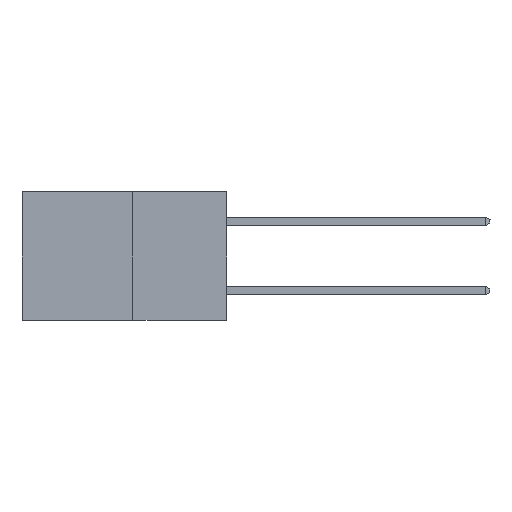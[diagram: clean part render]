
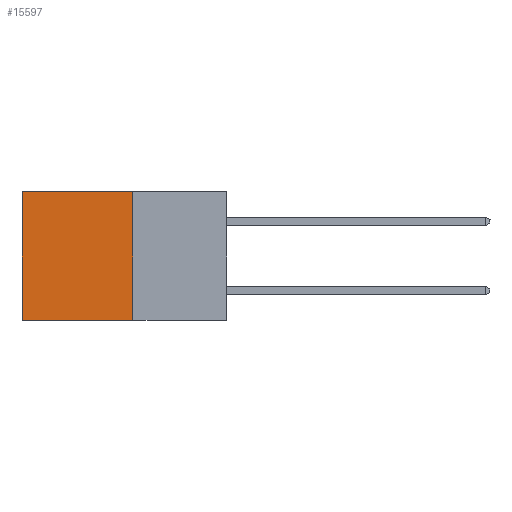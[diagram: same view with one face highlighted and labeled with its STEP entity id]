
A CAD part, left-side view. The second image highlights one B-rep face of the part: STEP entity #15597.
In plain terms, the highlighted planar face has unit normal (-1, 0, 0).
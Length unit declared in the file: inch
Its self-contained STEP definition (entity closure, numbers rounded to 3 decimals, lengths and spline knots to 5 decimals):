
#1082 = DIRECTION ( 'NONE',  ( 0., 1., 0. ) ) ;
#4852 = CARTESIAN_POINT ( 'NONE',  ( 0.277, 0.27, -0.37 ) ) ;
#4977 = CARTESIAN_POINT ( 'NONE',  ( 0.277, 0.27, -0.37 ) ) ;
#6089 = PLANE ( 'NONE',  #22583 ) ;
#6688 = VERTEX_POINT ( 'NONE', #24972 ) ;
#7414 = EDGE_CURVE ( 'NONE', #6688, #21558, #27898, .T. ) ;
#8300 = DIRECTION ( 'NONE',  ( 1., 0., 0. ) ) ;
#8343 = ORIENTED_EDGE ( 'NONE', *, *, #7414, .T. ) ;
#8910 = VECTOR ( 'NONE', #13236, 39.37008 ) ;
#9959 = EDGE_CURVE ( 'NONE', #21558, #11272, #15462, .T. ) ;
#11272 = VERTEX_POINT ( 'NONE', #15071 ) ;
#11439 = EDGE_CURVE ( 'NONE', #6688, #18386, #11996, .T. ) ;
#11572 = CARTESIAN_POINT ( 'NONE',  ( 0.277, 0.59, 0. ) ) ;
#11648 = DIRECTION ( 'NONE',  ( 0., 0., -1. ) ) ;
#11996 = LINE ( 'NONE', #4852, #17097 ) ;
#13236 = DIRECTION ( 'NONE',  ( 0., 0., -1. ) ) ;
#14269 = ORIENTED_EDGE ( 'NONE', *, *, #11439, .F. ) ;
#15071 = CARTESIAN_POINT ( 'NONE',  ( 0.277, 0.59, -0.37 ) ) ;
#15462 = LINE ( 'NONE', #24146, #8910 ) ;
#15550 = LINE ( 'NONE', #4977, #27225 ) ;
#15597 = ADVANCED_FACE ( 'NONE', ( #17437 ), #6089, .F. ) ;
#17097 = VECTOR ( 'NONE', #11648, 39.37008 ) ;
#17437 = FACE_OUTER_BOUND ( 'NONE', #17849, .T. ) ;
#17849 = EDGE_LOOP ( 'NONE', ( #21595, #21212, #14269, #8343 ) ) ;
#18386 = VERTEX_POINT ( 'NONE', #23468 ) ;
#18796 = EDGE_CURVE ( 'NONE', #18386, #11272, #15550, .T. ) ;
#20374 = DIRECTION ( 'NONE',  ( 0., 1., 0. ) ) ;
#20601 = CARTESIAN_POINT ( 'NONE',  ( 0.277, 0.27, 0. ) ) ;
#21212 = ORIENTED_EDGE ( 'NONE', *, *, #18796, .F. ) ;
#21478 = CARTESIAN_POINT ( 'NONE',  ( 0.277, 0.27, -0.37 ) ) ;
#21558 = VERTEX_POINT ( 'NONE', #11572 ) ;
#21595 = ORIENTED_EDGE ( 'NONE', *, *, #9959, .T. ) ;
#22583 = AXIS2_PLACEMENT_3D ( 'NONE', #21478, #8300, #23698 ) ;
#23468 = CARTESIAN_POINT ( 'NONE',  ( 0.277, 0.27, -0.37 ) ) ;
#23698 = DIRECTION ( 'NONE',  ( 0., 0., -1. ) ) ;
#24146 = CARTESIAN_POINT ( 'NONE',  ( 0.277, 0.59, -0.37 ) ) ;
#24972 = CARTESIAN_POINT ( 'NONE',  ( 0.277, 0.27, 0. ) ) ;
#27225 = VECTOR ( 'NONE', #20374, 39.37008 ) ;
#27233 = VECTOR ( 'NONE', #1082, 39.37008 ) ;
#27898 = LINE ( 'NONE', #20601, #27233 ) ;
